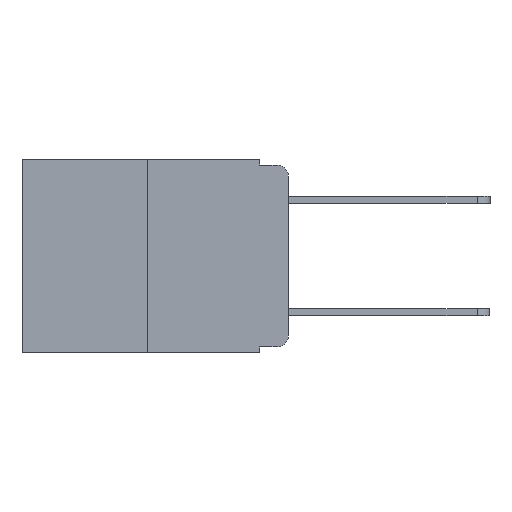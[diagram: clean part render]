
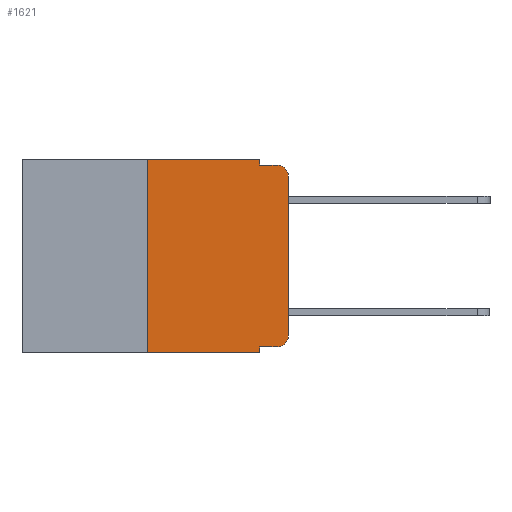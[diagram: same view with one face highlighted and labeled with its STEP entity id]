
A CAD part, left-side view. The second image highlights one B-rep face of the part: STEP entity #1621.
In plain terms, the highlighted planar face has unit normal (-1, 0, 0).
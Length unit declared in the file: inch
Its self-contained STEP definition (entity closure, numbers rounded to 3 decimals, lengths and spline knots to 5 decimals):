
#100 = ORIENTED_EDGE ( 'NONE', *, *, #11105, .T. ) ;
#120 = AXIS2_PLACEMENT_3D ( 'NONE', #7913, #551, #12865 ) ;
#551 = DIRECTION ( 'NONE',  ( 1., 0., 0. ) ) ;
#678 = ORIENTED_EDGE ( 'NONE', *, *, #2790, .F. ) ;
#788 = CARTESIAN_POINT ( 'NONE',  ( 0., 0., -0.313 ) ) ;
#1084 = ORIENTED_EDGE ( 'NONE', *, *, #15463, .F. ) ;
#1188 = CARTESIAN_POINT ( 'NONE',  ( 0., 0., -0.03 ) ) ;
#1193 = EDGE_CURVE ( 'NONE', #20160, #5852, #4054, .T. ) ;
#1621 = ADVANCED_FACE ( 'NONE', ( #19204 ), #20834, .F. ) ;
#1835 = ORIENTED_EDGE ( 'NONE', *, *, #19972, .T. ) ;
#2605 = EDGE_CURVE ( 'NONE', #3055, #5852, #13892, .T. ) ;
#2790 = EDGE_CURVE ( 'NONE', #17862, #11887, #18403, .T. ) ;
#2955 = CARTESIAN_POINT ( 'NONE',  ( 0., 0.25, 0. ) ) ;
#3055 = VERTEX_POINT ( 'NONE', #1188 ) ;
#3223 = LINE ( 'NONE', #17513, #16042 ) ;
#3781 = CARTESIAN_POINT ( 'NONE',  ( 0., 0.473, 0. ) ) ;
#3886 = VECTOR ( 'NONE', #6446, 39.37008 ) ;
#4054 = LINE ( 'NONE', #14389, #12926 ) ;
#4243 = AXIS2_PLACEMENT_3D ( 'NONE', #18518, #8816, #20088 ) ;
#4417 = LINE ( 'NONE', #20173, #21250 ) ;
#4465 = DIRECTION ( 'NONE',  ( 0., -1., 0. ) ) ;
#4516 = VECTOR ( 'NONE', #9907, 39.37008 ) ;
#4731 = CARTESIAN_POINT ( 'NONE',  ( 0., 0.02, -0.03 ) ) ;
#5020 = AXIS2_PLACEMENT_3D ( 'NONE', #4731, #16264, #6469 ) ;
#5100 = EDGE_CURVE ( 'NONE', #10805, #3055, #4417, .T. ) ;
#5852 = VERTEX_POINT ( 'NONE', #12089 ) ;
#6446 = DIRECTION ( 'NONE',  ( 0., 0., -1. ) ) ;
#6469 = DIRECTION ( 'NONE',  ( 0., 0., -1. ) ) ;
#6561 = CARTESIAN_POINT ( 'NONE',  ( 0., 0.473, -0.343 ) ) ;
#7219 = CARTESIAN_POINT ( 'NONE',  ( 0., 0.02, -0.333 ) ) ;
#7760 = VECTOR ( 'NONE', #9851, 39.37008 ) ;
#7913 = CARTESIAN_POINT ( 'NONE',  ( 0., 0.473, 0. ) ) ;
#8350 = EDGE_LOOP ( 'NONE', ( #12036, #12822, #13528, #15586, #678, #12270, #1835, #1084, #15133, #100 ) ) ;
#8538 = LINE ( 'NONE', #9806, #20898 ) ;
#8816 = DIRECTION ( 'NONE',  ( -1., 0., 0. ) ) ;
#9425 = DIRECTION ( 'NONE',  ( 0., -1., 0. ) ) ;
#9806 = CARTESIAN_POINT ( 'NONE',  ( 0., 0.25, 0. ) ) ;
#9851 = DIRECTION ( 'NONE',  ( 0., 0., -1. ) ) ;
#9907 = DIRECTION ( 'NONE',  ( 0., -1., 0. ) ) ;
#10805 = VERTEX_POINT ( 'NONE', #788 ) ;
#11105 = EDGE_CURVE ( 'NONE', #11149, #10805, #21284, .T. ) ;
#11149 = VERTEX_POINT ( 'NONE', #7219 ) ;
#11887 = VERTEX_POINT ( 'NONE', #15300 ) ;
#11966 = CARTESIAN_POINT ( 'NONE',  ( 0., 0.051, -0.01 ) ) ;
#12036 = ORIENTED_EDGE ( 'NONE', *, *, #5100, .T. ) ;
#12072 = VERTEX_POINT ( 'NONE', #22003 ) ;
#12089 = CARTESIAN_POINT ( 'NONE',  ( 0., 0.02, -0.01 ) ) ;
#12143 = LINE ( 'NONE', #19417, #7760 ) ;
#12192 = EDGE_CURVE ( 'NONE', #12072, #11149, #3223, .T. ) ;
#12270 = ORIENTED_EDGE ( 'NONE', *, *, #18654, .F. ) ;
#12822 = ORIENTED_EDGE ( 'NONE', *, *, #2605, .T. ) ;
#12865 = DIRECTION ( 'NONE',  ( 0., 0., -1. ) ) ;
#12926 = VECTOR ( 'NONE', #4465, 39.37008 ) ;
#13335 = LINE ( 'NONE', #6561, #4516 ) ;
#13528 = ORIENTED_EDGE ( 'NONE', *, *, #1193, .F. ) ;
#13892 = CIRCLE ( 'NONE', #5020, 0.02 ) ;
#14121 = VECTOR ( 'NONE', #15433, 39.37008 ) ;
#14389 = CARTESIAN_POINT ( 'NONE',  ( 0., 0.051, -0.01 ) ) ;
#15133 = ORIENTED_EDGE ( 'NONE', *, *, #12192, .T. ) ;
#15300 = CARTESIAN_POINT ( 'NONE',  ( 0., 0.051, 0. ) ) ;
#15433 = DIRECTION ( 'NONE',  ( 0., -1., 0. ) ) ;
#15463 = EDGE_CURVE ( 'NONE', #12072, #17947, #21285, .T. ) ;
#15482 = DIRECTION ( 'NONE',  ( 0., 0., 1. ) ) ;
#15586 = ORIENTED_EDGE ( 'NONE', *, *, #21830, .F. ) ;
#16042 = VECTOR ( 'NONE', #9425, 39.37008 ) ;
#16253 = CARTESIAN_POINT ( 'NONE',  ( 0., 0.051, 0. ) ) ;
#16264 = DIRECTION ( 'NONE',  ( -1., 0., 0. ) ) ;
#17513 = CARTESIAN_POINT ( 'NONE',  ( 0., 0.051, -0.333 ) ) ;
#17862 = VERTEX_POINT ( 'NONE', #2955 ) ;
#17947 = VERTEX_POINT ( 'NONE', #21207 ) ;
#18259 = CARTESIAN_POINT ( 'NONE',  ( 0., 0.25, -0.343 ) ) ;
#18403 = LINE ( 'NONE', #3781, #14121 ) ;
#18518 = CARTESIAN_POINT ( 'NONE',  ( 0., 0.02, -0.313 ) ) ;
#18654 = EDGE_CURVE ( 'NONE', #19397, #17862, #8538, .T. ) ;
#19204 = FACE_OUTER_BOUND ( 'NONE', #8350, .T. ) ;
#19397 = VERTEX_POINT ( 'NONE', #18259 ) ;
#19417 = CARTESIAN_POINT ( 'NONE',  ( 0., 0.051, 0. ) ) ;
#19438 = DIRECTION ( 'NONE',  ( 0., 0., 1. ) ) ;
#19972 = EDGE_CURVE ( 'NONE', #19397, #17947, #13335, .T. ) ;
#20088 = DIRECTION ( 'NONE',  ( 0., 0., -1. ) ) ;
#20160 = VERTEX_POINT ( 'NONE', #11966 ) ;
#20173 = CARTESIAN_POINT ( 'NONE',  ( 0., 0., 0. ) ) ;
#20834 = PLANE ( 'NONE',  #120 ) ;
#20898 = VECTOR ( 'NONE', #19438, 39.37008 ) ;
#21207 = CARTESIAN_POINT ( 'NONE',  ( 0., 0.051, -0.343 ) ) ;
#21250 = VECTOR ( 'NONE', #15482, 39.37008 ) ;
#21284 = CIRCLE ( 'NONE', #4243, 0.02 ) ;
#21285 = LINE ( 'NONE', #16253, #3886 ) ;
#21830 = EDGE_CURVE ( 'NONE', #11887, #20160, #12143, .T. ) ;
#22003 = CARTESIAN_POINT ( 'NONE',  ( 0., 0.051, -0.333 ) ) ;
